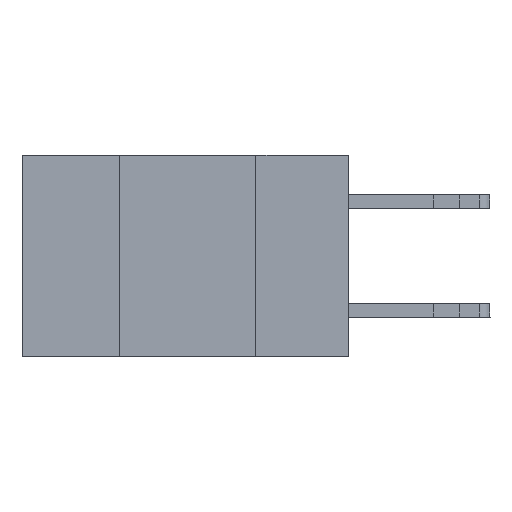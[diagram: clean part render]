
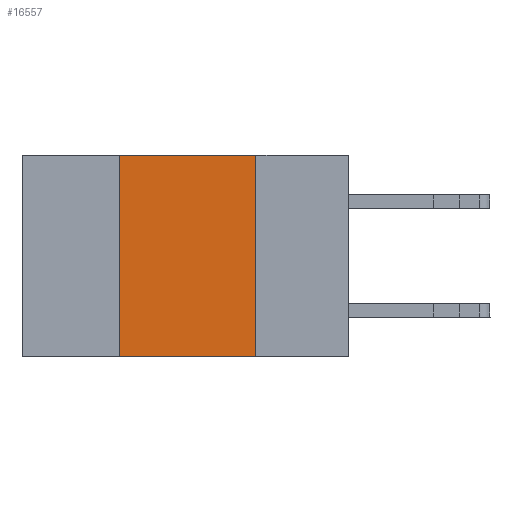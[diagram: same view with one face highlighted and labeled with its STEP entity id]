
A CAD part, left-side view. The second image highlights one B-rep face of the part: STEP entity #16557.
In plain terms, the highlighted planar face has unit normal (-1, 0, 0).
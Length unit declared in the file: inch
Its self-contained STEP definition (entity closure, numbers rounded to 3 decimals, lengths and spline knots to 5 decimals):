
#48 = AXIS2_PLACEMENT_3D ( 'NONE', #5339, #13847, #6780 ) ;
#51 = ORIENTED_EDGE ( 'NONE', *, *, #6077, .F. ) ;
#460 = VERTEX_POINT ( 'NONE', #9879 ) ;
#1078 = ORIENTED_EDGE ( 'NONE', *, *, #12297, .F. ) ;
#1102 = DIRECTION ( 'NONE',  ( 0., -1., 0. ) ) ;
#1280 = CARTESIAN_POINT ( 'NONE',  ( 0., 0.6, 0. ) ) ;
#1333 = LINE ( 'NONE', #1280, #4211 ) ;
#2374 = CARTESIAN_POINT ( 'NONE',  ( 0., 0.42, 0. ) ) ;
#3746 = EDGE_CURVE ( 'NONE', #14808, #16472, #6395, .T. ) ;
#4211 = VECTOR ( 'NONE', #1102, 39.37008 ) ;
#5339 = CARTESIAN_POINT ( 'NONE',  ( 0., 0.6, 0. ) ) ;
#5866 = VERTEX_POINT ( 'NONE', #8183 ) ;
#6077 = EDGE_CURVE ( 'NONE', #5866, #16472, #6791, .T. ) ;
#6395 = LINE ( 'NONE', #8163, #16836 ) ;
#6408 = CARTESIAN_POINT ( 'NONE',  ( 0., 0.17, -0.37 ) ) ;
#6780 = DIRECTION ( 'NONE',  ( 0., 0., -1. ) ) ;
#6791 = LINE ( 'NONE', #10854, #13883 ) ;
#8163 = CARTESIAN_POINT ( 'NONE',  ( 0., 0.6, -0.37 ) ) ;
#8183 = CARTESIAN_POINT ( 'NONE',  ( 0., 0.17, 0. ) ) ;
#9276 = PLANE ( 'NONE',  #48 ) ;
#9435 = FACE_OUTER_BOUND ( 'NONE', #12948, .T. ) ;
#9497 = DIRECTION ( 'NONE',  ( 0., 0., -1. ) ) ;
#9879 = CARTESIAN_POINT ( 'NONE',  ( 0., 0.42, 0. ) ) ;
#10370 = VECTOR ( 'NONE', #13408, 39.37008 ) ;
#10854 = CARTESIAN_POINT ( 'NONE',  ( 0., 0.17, 0. ) ) ;
#12297 = EDGE_CURVE ( 'NONE', #14808, #460, #17032, .T. ) ;
#12539 = ORIENTED_EDGE ( 'NONE', *, *, #13696, .F. ) ;
#12948 = EDGE_LOOP ( 'NONE', ( #51, #12539, #1078, #15568 ) ) ;
#13408 = DIRECTION ( 'NONE',  ( 0., 0., 1. ) ) ;
#13696 = EDGE_CURVE ( 'NONE', #460, #5866, #1333, .T. ) ;
#13847 = DIRECTION ( 'NONE',  ( 1., 0., 0. ) ) ;
#13883 = VECTOR ( 'NONE', #9497, 39.37008 ) ;
#14808 = VERTEX_POINT ( 'NONE', #14994 ) ;
#14994 = CARTESIAN_POINT ( 'NONE',  ( 0., 0.42, -0.37 ) ) ;
#15568 = ORIENTED_EDGE ( 'NONE', *, *, #3746, .T. ) ;
#16472 = VERTEX_POINT ( 'NONE', #6408 ) ;
#16557 = ADVANCED_FACE ( 'NONE', ( #9435 ), #9276, .F. ) ;
#16639 = DIRECTION ( 'NONE',  ( 0., -1., 0. ) ) ;
#16836 = VECTOR ( 'NONE', #16639, 39.37008 ) ;
#17032 = LINE ( 'NONE', #2374, #10370 ) ;
